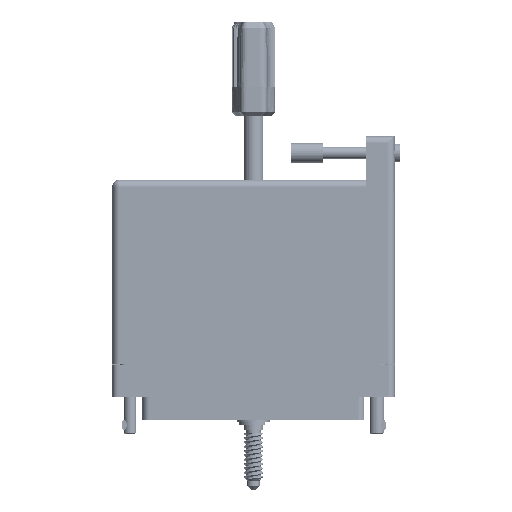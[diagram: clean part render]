
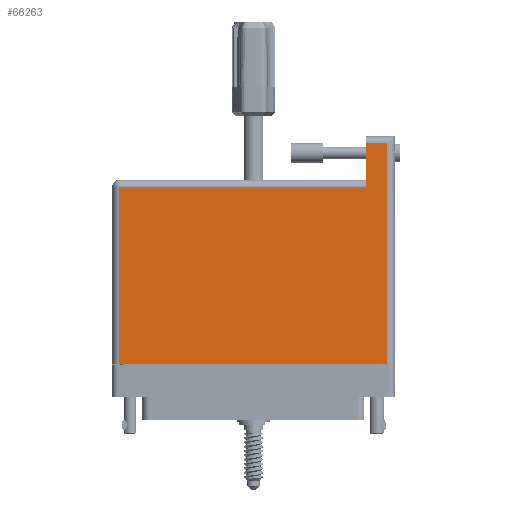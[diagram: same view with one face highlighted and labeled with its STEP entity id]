
A CAD part, front view. The second image highlights one B-rep face of the part: STEP entity #66263.
In plain terms, the highlighted face is planar.
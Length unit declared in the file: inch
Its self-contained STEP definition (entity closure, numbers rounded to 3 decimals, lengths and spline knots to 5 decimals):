
#3312 = LINE ( 'NONE', #96075, #47735 ) ;
#3816 = EDGE_CURVE ( 'NONE', #54505, #74757, #3312, .T. ) ;
#4002 = EDGE_CURVE ( 'NONE', #73233, #54505, #30131, .T. ) ;
#6133 = CARTESIAN_POINT ( 'NONE',  ( 1.079, 2.025, 0.617 ) ) ;
#6271 = CARTESIAN_POINT ( 'NONE',  ( 1.289, 2.095, 0.617 ) ) ;
#6600 = DIRECTION ( 'NONE',  ( 0., 1., 0. ) ) ;
#6680 = ORIENTED_EDGE ( 'NONE', *, *, #3816, .T. ) ;
#6872 = EDGE_LOOP ( 'NONE', ( #6680, #85953, #87530, #76797, #20419, #24089 ) ) ;
#15335 = DIRECTION ( 'NONE',  ( 0., 0., -1. ) ) ;
#17704 = CARTESIAN_POINT ( 'NONE',  ( 1.079, 2.095, 0.617 ) ) ;
#18686 = CARTESIAN_POINT ( 'NONE',  ( -1.289, -0.1, 0.617 ) ) ;
#20419 = ORIENTED_EDGE ( 'NONE', *, *, #63555, .T. ) ;
#20753 = VECTOR ( 'NONE', #32020, 39.37008 ) ;
#24089 = ORIENTED_EDGE ( 'NONE', *, *, #4002, .T. ) ;
#24530 = DIRECTION ( 'NONE',  ( -1., 0., 0. ) ) ;
#25545 = VECTOR ( 'NONE', #24530, 39.37008 ) ;
#25903 = CARTESIAN_POINT ( 'NONE',  ( -1.359, -0.1, 0.617 ) ) ;
#29942 = EDGE_CURVE ( 'NONE', #84688, #45277, #55062, .T. ) ;
#30131 = LINE ( 'NONE', #17704, #20753 ) ;
#32020 = DIRECTION ( 'NONE',  ( 0., -1., 0. ) ) ;
#37293 = CARTESIAN_POINT ( 'NONE',  ( -1.289, 1.605, 0.617 ) ) ;
#45028 = DIRECTION ( 'NONE',  ( -1., 0., 0. ) ) ;
#45277 = VERTEX_POINT ( 'NONE', #55786 ) ;
#47084 = CARTESIAN_POINT ( 'NONE',  ( 1.079, 1.605, 0.617 ) ) ;
#47504 = EDGE_CURVE ( 'NONE', #45277, #79527, #93250, .T. ) ;
#47735 = VECTOR ( 'NONE', #96704, 39.37008 ) ;
#51626 = AXIS2_PLACEMENT_3D ( 'NONE', #82519, #15335, #45028 ) ;
#54505 = VERTEX_POINT ( 'NONE', #47084 ) ;
#54614 = EDGE_CURVE ( 'NONE', #74757, #84688, #70540, .T. ) ;
#55062 = LINE ( 'NONE', #25903, #57421 ) ;
#55786 = CARTESIAN_POINT ( 'NONE',  ( 1.289, -0.1, 0.617 ) ) ;
#57421 = VECTOR ( 'NONE', #63063, 39.37008 ) ;
#61329 = CARTESIAN_POINT ( 'NONE',  ( -1.289, -0.1, 0.617 ) ) ;
#63063 = DIRECTION ( 'NONE',  ( 1., 0., 0. ) ) ;
#63555 = EDGE_CURVE ( 'NONE', #79527, #73233, #69890, .T. ) ;
#66263 = ADVANCED_FACE ( 'NONE', ( #75288 ), #89746, .F. ) ;
#69890 = LINE ( 'NONE', #75396, #25545 ) ;
#70540 = LINE ( 'NONE', #18686, #85688 ) ;
#71013 = VECTOR ( 'NONE', #6600, 39.37008 ) ;
#71478 = DIRECTION ( 'NONE',  ( 0., -1., 0. ) ) ;
#73233 = VERTEX_POINT ( 'NONE', #6133 ) ;
#74757 = VERTEX_POINT ( 'NONE', #37293 ) ;
#75288 = FACE_OUTER_BOUND ( 'NONE', #6872, .T. ) ;
#75396 = CARTESIAN_POINT ( 'NONE',  ( -1.359, 2.025, 0.617 ) ) ;
#76797 = ORIENTED_EDGE ( 'NONE', *, *, #47504, .T. ) ;
#79527 = VERTEX_POINT ( 'NONE', #94138 ) ;
#82519 = CARTESIAN_POINT ( 'NONE',  ( -1.359, 1.675, 0.617 ) ) ;
#84688 = VERTEX_POINT ( 'NONE', #61329 ) ;
#85688 = VECTOR ( 'NONE', #71478, 39.37008 ) ;
#85953 = ORIENTED_EDGE ( 'NONE', *, *, #54614, .T. ) ;
#87530 = ORIENTED_EDGE ( 'NONE', *, *, #29942, .T. ) ;
#89746 = PLANE ( 'NONE',  #51626 ) ;
#93250 = LINE ( 'NONE', #6271, #71013 ) ;
#94138 = CARTESIAN_POINT ( 'NONE',  ( 1.289, 2.025, 0.617 ) ) ;
#96075 = CARTESIAN_POINT ( 'NONE',  ( -1.359, 1.605, 0.617 ) ) ;
#96704 = DIRECTION ( 'NONE',  ( -1., 0., 0. ) ) ;
